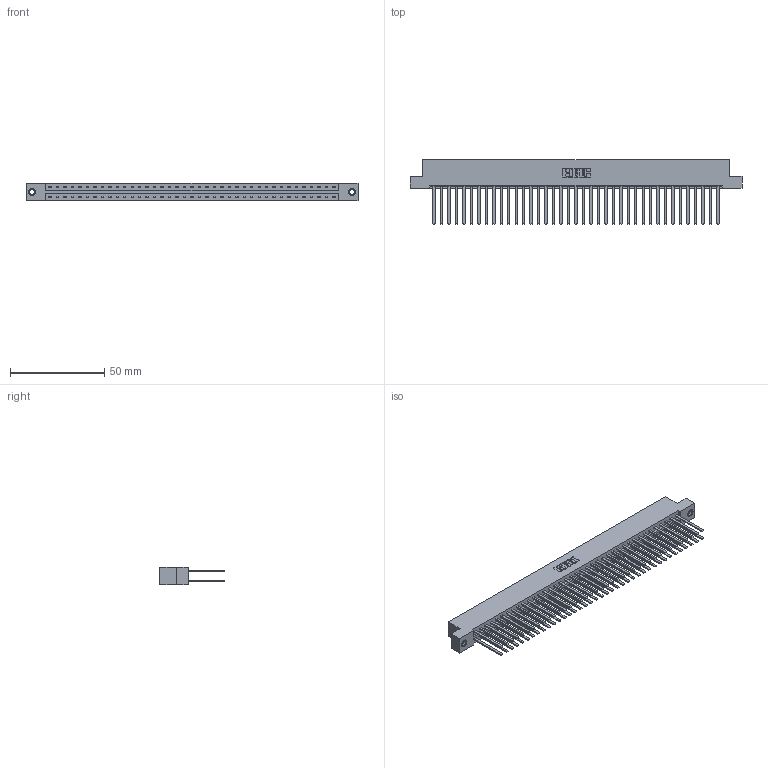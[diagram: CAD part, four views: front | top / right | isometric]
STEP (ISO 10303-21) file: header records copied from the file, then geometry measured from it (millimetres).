
FILE_DESCRIPTION (( 'STEP AP203' ), '1' );
FILE_NAME ('833-078-544-207.STEP', '2020-06-05T20:22:11', ( '' ), ( '' ), 'SwSTEP 2.0', 'SolidWorks 2020', '' );
FILE_SCHEMA (( 'CONFIG_CONTROL_DESIGN' ));
Length unit declared in the file: inch
Products named in the file (4): 833-078-544-207; 833 Part_Flush - .156 Dia - TI; 345-250-001_345-250-005-103; 345-292-001_345-293-144
Assembly tree (81 placements, depth 2):
  833-078-544-207
    833 Part_Flush - .156 Dia - TI
    345-292-001_345-293-144  x78
    345-250-001_345-250-005-103  x2
Bounding box: 176.07 x 34.3 x 9.4 mm (x, y, z)
Volume: 19027.9 mm3; surface area: 26018.1 mm2
Topology: 81 solids, 81 shells, 3762 faces, 11133 edges, 7310 vertices
Faces by surface type: plane 2598, cylinder 1148, cone 12, torus 4
Entity records: 26480 total; most frequent: CARTESIAN_POINT 4373, ORIENTED_EDGE 4302, DIRECTION 3769, EDGE_CURVE 2151, LINE 2007, VECTOR 2007, VERTEX_POINT 1428, AXIS2_PLACEMENT_3D 881
